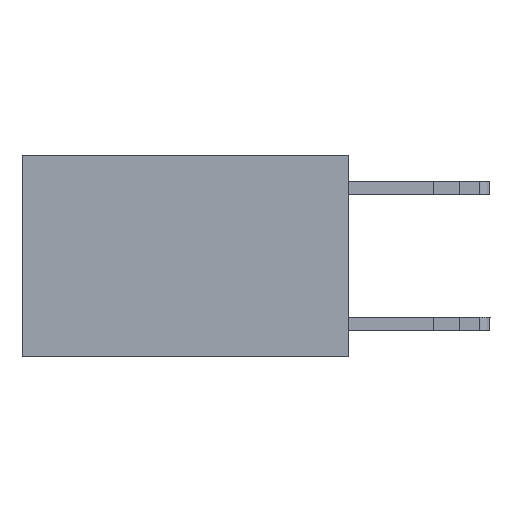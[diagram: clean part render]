
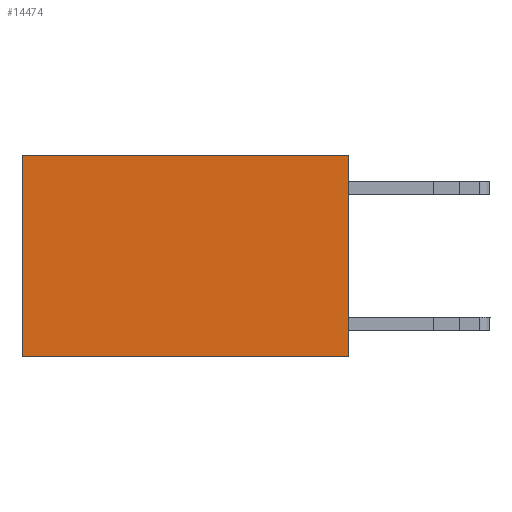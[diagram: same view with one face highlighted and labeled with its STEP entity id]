
A CAD part, left-side view. The second image highlights one B-rep face of the part: STEP entity #14474.
In plain terms, the highlighted planar face has unit normal (-1, 0, 0).
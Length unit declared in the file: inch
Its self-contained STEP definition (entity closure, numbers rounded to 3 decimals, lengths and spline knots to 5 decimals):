
#22 = EDGE_LOOP ( 'NONE', ( #5162, #14942, #1852, #8007 ) ) ;
#1205 = DIRECTION ( 'NONE',  ( 0., 0., -1. ) ) ;
#1852 = ORIENTED_EDGE ( 'NONE', *, *, #3552, .F. ) ;
#3552 = EDGE_CURVE ( 'NONE', #22952, #19550, #3868, .T. ) ;
#3868 = LINE ( 'NONE', #19566, #23563 ) ;
#4959 = DIRECTION ( 'NONE',  ( 0., 1., 0. ) ) ;
#5162 = ORIENTED_EDGE ( 'NONE', *, *, #21592, .T. ) ;
#6227 = VERTEX_POINT ( 'NONE', #6545 ) ;
#6446 = CARTESIAN_POINT ( 'NONE',  ( 0.2625, 0.6, -0.37 ) ) ;
#6545 = CARTESIAN_POINT ( 'NONE',  ( 0.2625, 0.6, 0. ) ) ;
#6876 = CARTESIAN_POINT ( 'NONE',  ( 0.2625, 0., -0.37 ) ) ;
#7261 = PLANE ( 'NONE',  #15468 ) ;
#7407 = VECTOR ( 'NONE', #1205, 39.37008 ) ;
#8007 = ORIENTED_EDGE ( 'NONE', *, *, #10725, .T. ) ;
#8776 = LINE ( 'NONE', #13001, #17924 ) ;
#8813 = VERTEX_POINT ( 'NONE', #6446 ) ;
#8936 = CARTESIAN_POINT ( 'NONE',  ( 0.2625, 0., 0. ) ) ;
#10497 = EDGE_CURVE ( 'NONE', #19550, #8813, #18279, .T. ) ;
#10725 = EDGE_CURVE ( 'NONE', #22952, #6227, #8776, .T. ) ;
#10949 = CARTESIAN_POINT ( 'NONE',  ( 0.2625, 0., 0. ) ) ;
#11900 = DIRECTION ( 'NONE',  ( 0., 0., -1. ) ) ;
#13001 = CARTESIAN_POINT ( 'NONE',  ( 0.2625, 0., 0. ) ) ;
#13346 = CARTESIAN_POINT ( 'NONE',  ( 0.2625, 0.6, 0. ) ) ;
#13463 = DIRECTION ( 'NONE',  ( 0., 0., -1. ) ) ;
#14474 = ADVANCED_FACE ( 'NONE', ( #19390 ), #7261, .F. ) ;
#14942 = ORIENTED_EDGE ( 'NONE', *, *, #10497, .F. ) ;
#15468 = AXIS2_PLACEMENT_3D ( 'NONE', #10949, #17152, #13463 ) ;
#17152 = DIRECTION ( 'NONE',  ( 1., 0., 0. ) ) ;
#17514 = VECTOR ( 'NONE', #24339, 39.37008 ) ;
#17924 = VECTOR ( 'NONE', #4959, 39.37008 ) ;
#18279 = LINE ( 'NONE', #20260, #17514 ) ;
#19390 = FACE_OUTER_BOUND ( 'NONE', #22, .T. ) ;
#19550 = VERTEX_POINT ( 'NONE', #6876 ) ;
#19566 = CARTESIAN_POINT ( 'NONE',  ( 0.2625, 0., 0. ) ) ;
#20260 = CARTESIAN_POINT ( 'NONE',  ( 0.2625, 0., -0.37 ) ) ;
#21378 = LINE ( 'NONE', #13346, #7407 ) ;
#21592 = EDGE_CURVE ( 'NONE', #6227, #8813, #21378, .T. ) ;
#22952 = VERTEX_POINT ( 'NONE', #8936 ) ;
#23563 = VECTOR ( 'NONE', #11900, 39.37008 ) ;
#24339 = DIRECTION ( 'NONE',  ( 0., 1., 0. ) ) ;
